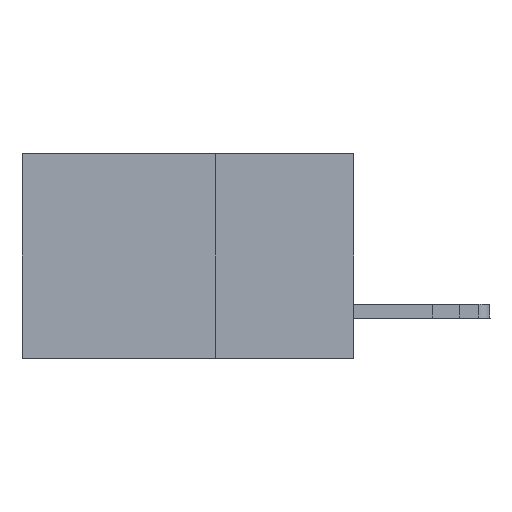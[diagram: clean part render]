
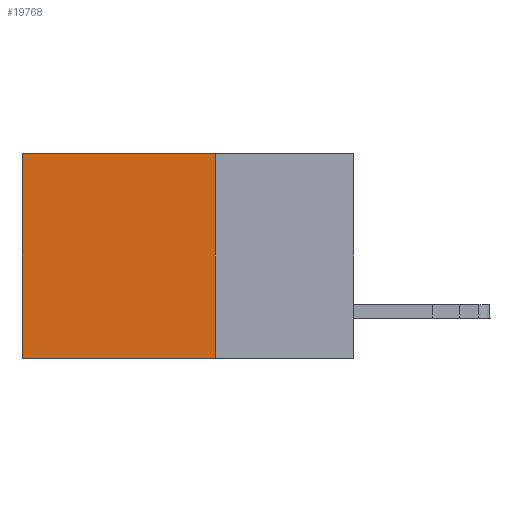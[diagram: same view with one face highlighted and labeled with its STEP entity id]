
A CAD part, left-side view. The second image highlights one B-rep face of the part: STEP entity #19768.
In plain terms, the highlighted planar face has unit normal (-1, 0, 0).
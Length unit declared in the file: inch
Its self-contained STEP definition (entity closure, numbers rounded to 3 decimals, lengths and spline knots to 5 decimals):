
#640 = DIRECTION ( 'NONE',  ( 0., 1., 0. ) ) ;
#1067 = DIRECTION ( 'NONE',  ( 0., 1., 0. ) ) ;
#1102 = FACE_OUTER_BOUND ( 'NONE', #7531, .T. ) ;
#1890 = CARTESIAN_POINT ( 'NONE',  ( 0.2875, 0.6, -0.37 ) ) ;
#2169 = VECTOR ( 'NONE', #1067, 39.37008 ) ;
#2287 = VECTOR ( 'NONE', #640, 39.37008 ) ;
#3712 = ORIENTED_EDGE ( 'NONE', *, *, #15411, .T. ) ;
#3973 = AXIS2_PLACEMENT_3D ( 'NONE', #21855, #10084, #23800 ) ;
#4013 = EDGE_CURVE ( 'NONE', #24622, #18845, #4324, .T. ) ;
#4292 = DIRECTION ( 'NONE',  ( 0., 0., -1. ) ) ;
#4324 = LINE ( 'NONE', #21861, #18691 ) ;
#7531 = EDGE_LOOP ( 'NONE', ( #17056, #18150, #9330, #3712 ) ) ;
#7759 = CARTESIAN_POINT ( 'NONE',  ( 0.2875, 0.6, 0. ) ) ;
#8123 = LINE ( 'NONE', #7759, #9348 ) ;
#9330 = ORIENTED_EDGE ( 'NONE', *, *, #4013, .F. ) ;
#9348 = VECTOR ( 'NONE', #23428, 39.37008 ) ;
#10084 = DIRECTION ( 'NONE',  ( 1., 0., 0. ) ) ;
#11962 = CARTESIAN_POINT ( 'NONE',  ( 0.2875, 0.25, 0. ) ) ;
#12021 = VERTEX_POINT ( 'NONE', #16508 ) ;
#12332 = CARTESIAN_POINT ( 'NONE',  ( 0.2875, 0.25, 0. ) ) ;
#12549 = LINE ( 'NONE', #20561, #2169 ) ;
#13942 = PLANE ( 'NONE',  #3973 ) ;
#14937 = CARTESIAN_POINT ( 'NONE',  ( 0.2875, 0.25, -0.37 ) ) ;
#15411 = EDGE_CURVE ( 'NONE', #24622, #12021, #17270, .T. ) ;
#16508 = CARTESIAN_POINT ( 'NONE',  ( 0.2875, 0.6, 0. ) ) ;
#17056 = ORIENTED_EDGE ( 'NONE', *, *, #19052, .T. ) ;
#17270 = LINE ( 'NONE', #12332, #2287 ) ;
#18150 = ORIENTED_EDGE ( 'NONE', *, *, #22722, .F. ) ;
#18691 = VECTOR ( 'NONE', #4292, 39.37008 ) ;
#18845 = VERTEX_POINT ( 'NONE', #14937 ) ;
#19052 = EDGE_CURVE ( 'NONE', #12021, #24498, #8123, .T. ) ;
#19768 = ADVANCED_FACE ( 'NONE', ( #1102 ), #13942, .F. ) ;
#20561 = CARTESIAN_POINT ( 'NONE',  ( 0.2875, 0.25, -0.37 ) ) ;
#21855 = CARTESIAN_POINT ( 'NONE',  ( 0.2875, 0.25, 0. ) ) ;
#21861 = CARTESIAN_POINT ( 'NONE',  ( 0.2875, 0.25, 0. ) ) ;
#22722 = EDGE_CURVE ( 'NONE', #18845, #24498, #12549, .T. ) ;
#23428 = DIRECTION ( 'NONE',  ( 0., 0., -1. ) ) ;
#23800 = DIRECTION ( 'NONE',  ( 0., 0., -1. ) ) ;
#24498 = VERTEX_POINT ( 'NONE', #1890 ) ;
#24622 = VERTEX_POINT ( 'NONE', #11962 ) ;
